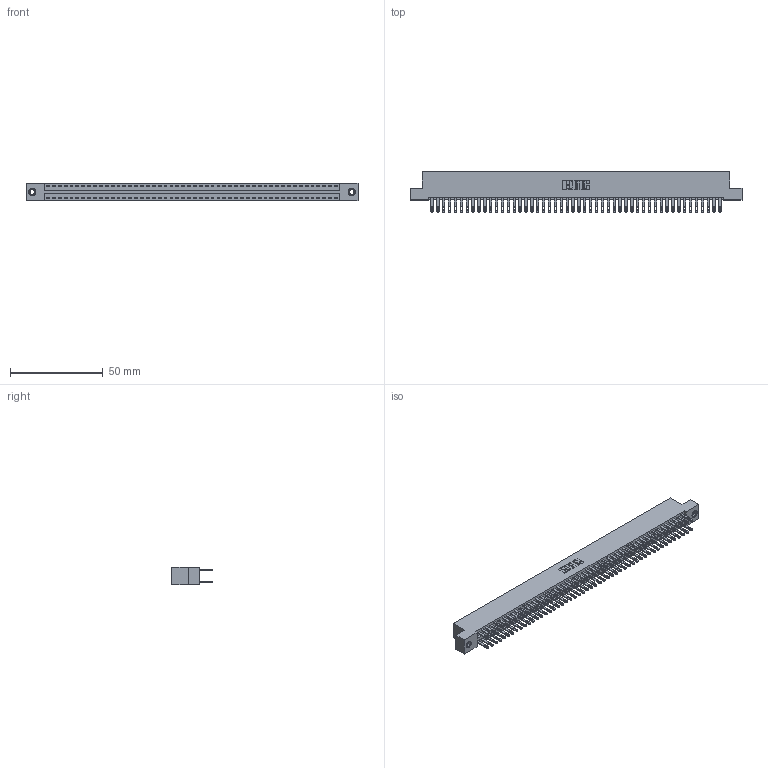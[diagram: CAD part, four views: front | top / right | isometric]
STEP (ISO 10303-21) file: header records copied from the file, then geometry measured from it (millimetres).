
FILE_DESCRIPTION (( 'STEP AP203' ), '1' );
FILE_NAME ('346-100-500-207.STEP', '2018-08-30T10:02:15', ( '' ), ( '' ), 'SwSTEP 2.0', 'SolidWorks 2016', '' );
FILE_SCHEMA (( 'CONFIG_CONTROL_DESIGN' ));
Length unit declared in the file: inch
Products named in the file (4): 346 Part_Flush Mounting Lugs - 0.156 Dia-TI; 345-292-001_345-293-100; 345-250-001_345-250-005-103; 346-100-500-207
Assembly tree (103 placements, depth 2):
  346-100-500-207
    346 Part_Flush Mounting Lugs - 0.156 Dia-TI
    345-292-001_345-293-100  x100
    345-250-001_345-250-005-103  x2
Bounding box: 179.32 x 21.84 x 9.4 mm (x, y, z)
Volume: 17840.5 mm3; surface area: 25729.1 mm2
Topology: 103 solids, 103 shells, 4982 faces, 15165 edges, 10102 vertices
Faces by surface type: plane 3008, cylinder 1958, cone 12, torus 4
Entity records: 32670 total; most frequent: CARTESIAN_POINT 5355, ORIENTED_EDGE 5282, DIRECTION 4799, EDGE_CURVE 2641, LINE 2285, VECTOR 2285, VERTEX_POINT 1756, AXIS2_PLACEMENT_3D 1257
